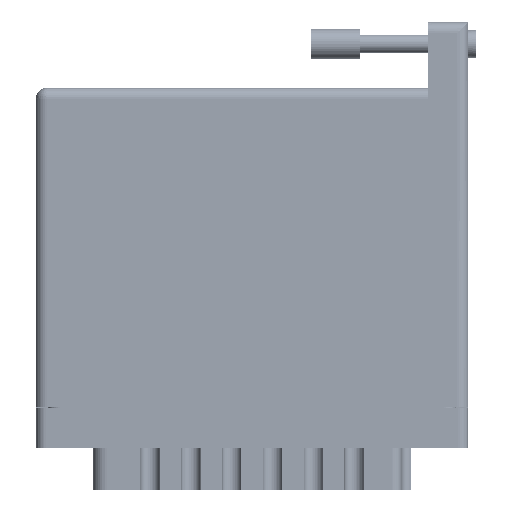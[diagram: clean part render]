
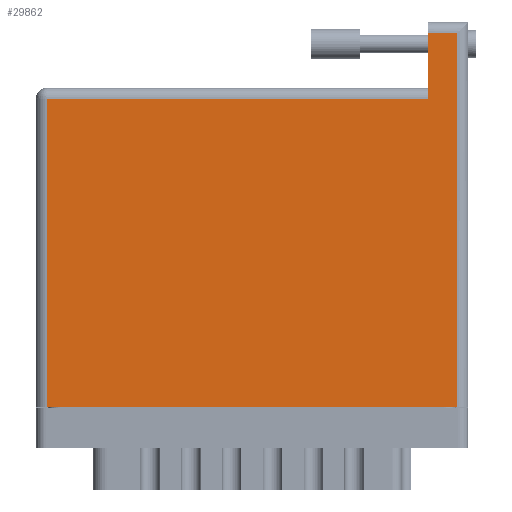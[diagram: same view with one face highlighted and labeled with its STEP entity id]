
A CAD part, front view. The second image highlights one B-rep face of the part: STEP entity #29862.
In plain terms, the highlighted face is planar.
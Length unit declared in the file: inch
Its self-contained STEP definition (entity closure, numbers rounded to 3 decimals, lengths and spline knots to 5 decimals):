
#2025 = EDGE_LOOP ( 'NONE', ( #13340, #32668, #24540, #37673, #36813, #92019 ) ) ;
#3563 = EDGE_CURVE ( 'NONE', #11288, #89959, #27585, .T. ) ;
#7208 = FACE_OUTER_BOUND ( 'NONE', #2025, .T. ) ;
#7917 = LINE ( 'NONE', #38289, #78398 ) ;
#9135 = DIRECTION ( 'NONE',  ( 0., -1., 0. ) ) ;
#11288 = VERTEX_POINT ( 'NONE', #80051 ) ;
#12211 = CARTESIAN_POINT ( 'NONE',  ( 2.685, 0., 0. ) ) ;
#13138 = LINE ( 'NONE', #57245, #26672 ) ;
#13340 = ORIENTED_EDGE ( 'NONE', *, *, #40430, .T. ) ;
#17248 = LINE ( 'NONE', #90379, #29550 ) ;
#18408 = CARTESIAN_POINT ( 'NONE',  ( 2.499, 1.96, 0. ) ) ;
#19781 = VECTOR ( 'NONE', #50402, 39.37008 ) ;
#21743 = CARTESIAN_POINT ( 'NONE',  ( 0., 0., 0. ) ) ;
#23244 = VERTEX_POINT ( 'NONE', #44842 ) ;
#24044 = DIRECTION ( 'NONE',  ( -1., 0., 0. ) ) ;
#24540 = ORIENTED_EDGE ( 'NONE', *, *, #25343, .T. ) ;
#25343 = EDGE_CURVE ( 'NONE', #55380, #11288, #51685, .T. ) ;
#26672 = VECTOR ( 'NONE', #78468, 39.37008 ) ;
#27585 = LINE ( 'NONE', #21743, #30881 ) ;
#29550 = VECTOR ( 'NONE', #55354, 39.37008 ) ;
#29862 = ADVANCED_FACE ( 'NONE', ( #7208 ), #60296, .F. ) ;
#30881 = VECTOR ( 'NONE', #43047, 39.37008 ) ;
#30899 = CARTESIAN_POINT ( 'NONE',  ( 0., 2.03, 0. ) ) ;
#32668 = ORIENTED_EDGE ( 'NONE', *, *, #51916, .T. ) ;
#36245 = DIRECTION ( 'NONE',  ( 0., -1., 0. ) ) ;
#36813 = ORIENTED_EDGE ( 'NONE', *, *, #76546, .T. ) ;
#37673 = ORIENTED_EDGE ( 'NONE', *, *, #3563, .T. ) ;
#38289 = CARTESIAN_POINT ( 'NONE',  ( 2.499, 2.45, 0. ) ) ;
#40430 = EDGE_CURVE ( 'NONE', #62201, #76853, #7917, .T. ) ;
#42780 = CARTESIAN_POINT ( 'NONE',  ( 0.07, 1.96, 0. ) ) ;
#43047 = DIRECTION ( 'NONE',  ( 1., 0., 0. ) ) ;
#43989 = AXIS2_PLACEMENT_3D ( 'NONE', #30899, #80950, #24044 ) ;
#44842 = CARTESIAN_POINT ( 'NONE',  ( 2.685, 2.38, 0. ) ) ;
#50402 = DIRECTION ( 'NONE',  ( 0., 1., 0. ) ) ;
#51685 = LINE ( 'NONE', #79088, #91993 ) ;
#51916 = EDGE_CURVE ( 'NONE', #76853, #55380, #17248, .T. ) ;
#53847 = LINE ( 'NONE', #56379, #19781 ) ;
#55354 = DIRECTION ( 'NONE',  ( -1., 0., 0. ) ) ;
#55380 = VERTEX_POINT ( 'NONE', #42780 ) ;
#56379 = CARTESIAN_POINT ( 'NONE',  ( 2.685, 2.45, 0. ) ) ;
#57245 = CARTESIAN_POINT ( 'NONE',  ( 0., 2.38, 0. ) ) ;
#60296 = PLANE ( 'NONE',  #43989 ) ;
#62201 = VERTEX_POINT ( 'NONE', #79985 ) ;
#67222 = EDGE_CURVE ( 'NONE', #23244, #62201, #13138, .T. ) ;
#76546 = EDGE_CURVE ( 'NONE', #89959, #23244, #53847, .T. ) ;
#76853 = VERTEX_POINT ( 'NONE', #18408 ) ;
#78398 = VECTOR ( 'NONE', #9135, 39.37008 ) ;
#78468 = DIRECTION ( 'NONE',  ( -1., 0., 0. ) ) ;
#79088 = CARTESIAN_POINT ( 'NONE',  ( 0.07, 0., 0. ) ) ;
#79985 = CARTESIAN_POINT ( 'NONE',  ( 2.499, 2.38, 0. ) ) ;
#80051 = CARTESIAN_POINT ( 'NONE',  ( 0.07, 0., 0. ) ) ;
#80950 = DIRECTION ( 'NONE',  ( 0., 0., -1. ) ) ;
#89959 = VERTEX_POINT ( 'NONE', #12211 ) ;
#90379 = CARTESIAN_POINT ( 'NONE',  ( 0., 1.96, 0. ) ) ;
#91993 = VECTOR ( 'NONE', #36245, 39.37008 ) ;
#92019 = ORIENTED_EDGE ( 'NONE', *, *, #67222, .T. ) ;
